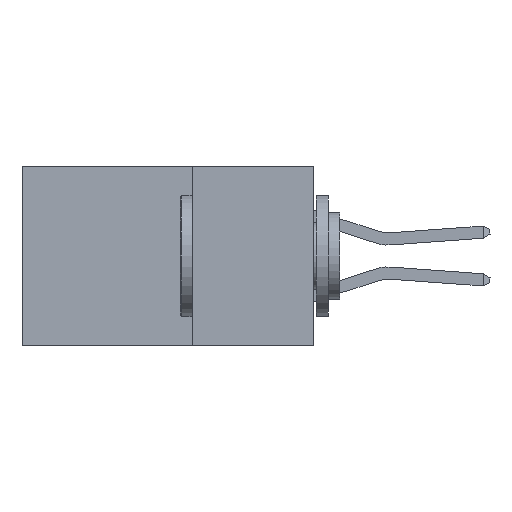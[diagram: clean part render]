
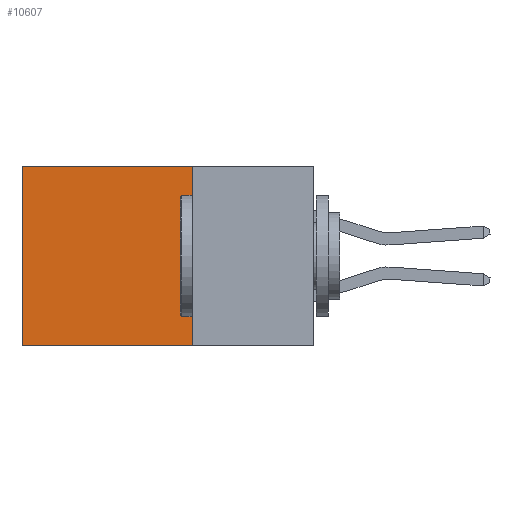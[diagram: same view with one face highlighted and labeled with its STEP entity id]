
A CAD part, left-side view. The second image highlights one B-rep face of the part: STEP entity #10607.
In plain terms, the highlighted planar face has unit normal (-1, 0, 0).
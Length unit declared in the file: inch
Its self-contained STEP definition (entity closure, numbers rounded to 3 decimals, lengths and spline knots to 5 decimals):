
#1247 = EDGE_CURVE ( 'NONE', #23257, #2809, #26286, .T. ) ;
#1481 = CARTESIAN_POINT ( 'NONE',  ( 0.2875, 0.25, 0. ) ) ;
#2508 = ORIENTED_EDGE ( 'NONE', *, *, #8663, .T. ) ;
#2809 = VERTEX_POINT ( 'NONE', #7815 ) ;
#3331 = VECTOR ( 'NONE', #24143, 39.37008 ) ;
#5332 = DIRECTION ( 'NONE',  ( 0., 1., 0. ) ) ;
#5419 = LINE ( 'NONE', #21943, #3331 ) ;
#5444 = ORIENTED_EDGE ( 'NONE', *, *, #1247, .F. ) ;
#5809 = DIRECTION ( 'NONE',  ( 0., 0., -1. ) ) ;
#6138 = LINE ( 'NONE', #14972, #27542 ) ;
#7810 = DIRECTION ( 'NONE',  ( 0., 0., -1. ) ) ;
#7815 = CARTESIAN_POINT ( 'NONE',  ( 0.2875, 0.6, -0.37 ) ) ;
#8663 = EDGE_CURVE ( 'NONE', #17157, #2809, #6138, .T. ) ;
#9663 = ORIENTED_EDGE ( 'NONE', *, *, #28417, .F. ) ;
#10240 = ORIENTED_EDGE ( 'NONE', *, *, #23955, .T. ) ;
#10264 = LINE ( 'NONE', #19059, #21651 ) ;
#10607 = ADVANCED_FACE ( 'NONE', ( #16058 ), #18747, .F. ) ;
#10903 = AXIS2_PLACEMENT_3D ( 'NONE', #1481, #25562, #7810 ) ;
#12853 = CARTESIAN_POINT ( 'NONE',  ( 0.2875, 0.25, 0. ) ) ;
#13951 = DIRECTION ( 'NONE',  ( 0., 0., -1. ) ) ;
#14972 = CARTESIAN_POINT ( 'NONE',  ( 0.2875, 0.6, 0. ) ) ;
#16056 = CARTESIAN_POINT ( 'NONE',  ( 0.2875, 0.6, 0. ) ) ;
#16058 = FACE_OUTER_BOUND ( 'NONE', #24435, .T. ) ;
#17157 = VERTEX_POINT ( 'NONE', #16056 ) ;
#18747 = PLANE ( 'NONE',  #10903 ) ;
#18951 = CARTESIAN_POINT ( 'NONE',  ( 0.2875, 0.25, -0.37 ) ) ;
#19059 = CARTESIAN_POINT ( 'NONE',  ( 0.2875, 0.25, 0. ) ) ;
#20439 = VECTOR ( 'NONE', #5332, 39.37008 ) ;
#21651 = VECTOR ( 'NONE', #5809, 39.37008 ) ;
#21943 = CARTESIAN_POINT ( 'NONE',  ( 0.2875, 0.25, 0. ) ) ;
#23257 = VERTEX_POINT ( 'NONE', #23296 ) ;
#23296 = CARTESIAN_POINT ( 'NONE',  ( 0.2875, 0.25, -0.37 ) ) ;
#23955 = EDGE_CURVE ( 'NONE', #27183, #17157, #5419, .T. ) ;
#24143 = DIRECTION ( 'NONE',  ( 0., 1., 0. ) ) ;
#24435 = EDGE_LOOP ( 'NONE', ( #2508, #5444, #9663, #10240 ) ) ;
#25562 = DIRECTION ( 'NONE',  ( 1., 0., 0. ) ) ;
#26286 = LINE ( 'NONE', #18951, #20439 ) ;
#27183 = VERTEX_POINT ( 'NONE', #12853 ) ;
#27542 = VECTOR ( 'NONE', #13951, 39.37008 ) ;
#28417 = EDGE_CURVE ( 'NONE', #27183, #23257, #10264, .T. ) ;
